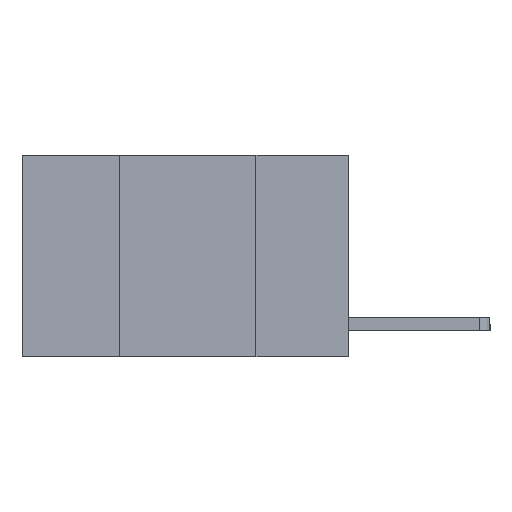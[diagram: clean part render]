
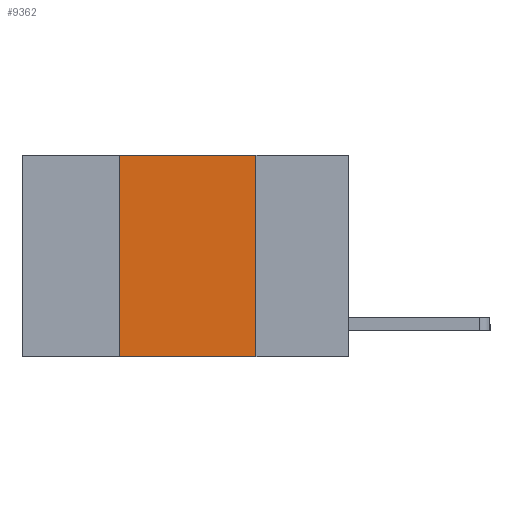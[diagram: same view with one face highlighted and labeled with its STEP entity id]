
A CAD part, left-side view. The second image highlights one B-rep face of the part: STEP entity #9362.
In plain terms, the highlighted planar face has unit normal (-1, 0, 0).
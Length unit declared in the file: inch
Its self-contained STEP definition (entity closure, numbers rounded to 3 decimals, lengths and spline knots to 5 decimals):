
#107 = ORIENTED_EDGE ( 'NONE', *, *, #237, .F. ) ;
#198 = EDGE_CURVE ( 'NONE', #2243, #4829, #8074, .T. ) ;
#237 = EDGE_CURVE ( 'NONE', #8215, #4869, #3297, .T. ) ;
#459 = EDGE_CURVE ( 'NONE', #2243, #4869, #3906, .T. ) ;
#663 = DIRECTION ( 'NONE',  ( 0., 0., 1. ) ) ;
#725 = CARTESIAN_POINT ( 'NONE',  ( 0., 0.42, 0. ) ) ;
#1055 = CARTESIAN_POINT ( 'NONE',  ( 0., 0.17, -0.37 ) ) ;
#1220 = CARTESIAN_POINT ( 'NONE',  ( 0., 0.6, -0.37 ) ) ;
#1353 = VECTOR ( 'NONE', #2596, 39.37008 ) ;
#1508 = CARTESIAN_POINT ( 'NONE',  ( 0., 0.42, -0.37 ) ) ;
#1581 = DIRECTION ( 'NONE',  ( 0., -1., 0. ) ) ;
#2139 = DIRECTION ( 'NONE',  ( 0., 0., -1. ) ) ;
#2243 = VERTEX_POINT ( 'NONE', #1508 ) ;
#2351 = ORIENTED_EDGE ( 'NONE', *, *, #198, .F. ) ;
#2596 = DIRECTION ( 'NONE',  ( 0., 0., -1. ) ) ;
#3074 = CARTESIAN_POINT ( 'NONE',  ( 0., 0.6, 0. ) ) ;
#3133 = CARTESIAN_POINT ( 'NONE',  ( 0., 0.42, 0. ) ) ;
#3297 = LINE ( 'NONE', #5002, #1353 ) ;
#3571 = ORIENTED_EDGE ( 'NONE', *, *, #459, .T. ) ;
#3631 = VECTOR ( 'NONE', #6418, 39.37008 ) ;
#3906 = LINE ( 'NONE', #1220, #3631 ) ;
#4431 = CARTESIAN_POINT ( 'NONE',  ( 0., 0.6, 0. ) ) ;
#4466 = AXIS2_PLACEMENT_3D ( 'NONE', #4431, #6106, #2139 ) ;
#4489 = FACE_OUTER_BOUND ( 'NONE', #9015, .T. ) ;
#4829 = VERTEX_POINT ( 'NONE', #3133 ) ;
#4869 = VERTEX_POINT ( 'NONE', #1055 ) ;
#5002 = CARTESIAN_POINT ( 'NONE',  ( 0., 0.17, 0. ) ) ;
#6106 = DIRECTION ( 'NONE',  ( 1., 0., 0. ) ) ;
#6418 = DIRECTION ( 'NONE',  ( 0., -1., 0. ) ) ;
#7012 = VECTOR ( 'NONE', #1581, 39.37008 ) ;
#8074 = LINE ( 'NONE', #725, #8191 ) ;
#8191 = VECTOR ( 'NONE', #663, 39.37008 ) ;
#8215 = VERTEX_POINT ( 'NONE', #8924 ) ;
#8924 = CARTESIAN_POINT ( 'NONE',  ( 0., 0.17, 0. ) ) ;
#9015 = EDGE_LOOP ( 'NONE', ( #107, #10561, #2351, #3571 ) ) ;
#9362 = ADVANCED_FACE ( 'NONE', ( #4489 ), #10237, .F. ) ;
#9920 = EDGE_CURVE ( 'NONE', #4829, #8215, #10423, .T. ) ;
#10237 = PLANE ( 'NONE',  #4466 ) ;
#10423 = LINE ( 'NONE', #3074, #7012 ) ;
#10561 = ORIENTED_EDGE ( 'NONE', *, *, #9920, .F. ) ;
